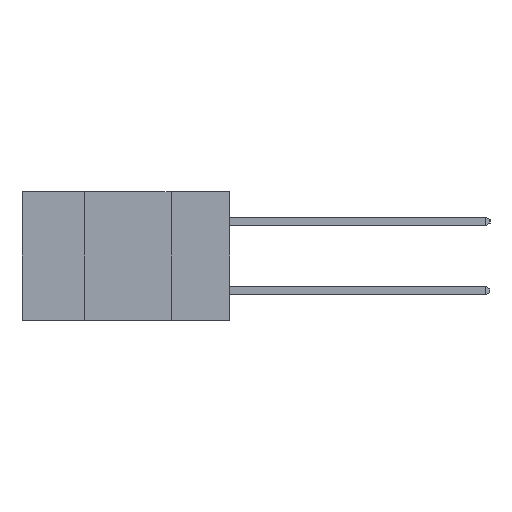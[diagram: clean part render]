
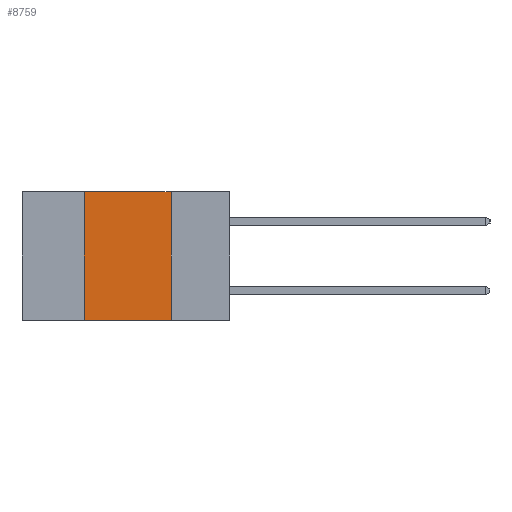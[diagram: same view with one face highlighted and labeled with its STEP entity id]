
A CAD part, left-side view. The second image highlights one B-rep face of the part: STEP entity #8759.
In plain terms, the highlighted planar face has unit normal (-1, 0, 0).
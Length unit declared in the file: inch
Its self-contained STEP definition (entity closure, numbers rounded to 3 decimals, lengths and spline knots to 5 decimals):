
#1374 = EDGE_CURVE ( 'NONE', #15556, #14151, #3866, .T. ) ;
#1461 = DIRECTION ( 'NONE',  ( 0., -1., 0. ) ) ;
#1556 = FACE_OUTER_BOUND ( 'NONE', #8169, .T. ) ;
#2728 = CARTESIAN_POINT ( 'NONE',  ( 0., 0.6, 0. ) ) ;
#2753 = VERTEX_POINT ( 'NONE', #3035 ) ;
#3035 = CARTESIAN_POINT ( 'NONE',  ( 0., 0.42, -0.37 ) ) ;
#3044 = EDGE_CURVE ( 'NONE', #2753, #14151, #6823, .T. ) ;
#3290 = PLANE ( 'NONE',  #7821 ) ;
#3391 = DIRECTION ( 'NONE',  ( 0., -1., 0. ) ) ;
#3539 = VECTOR ( 'NONE', #3391, 39.37008 ) ;
#3866 = LINE ( 'NONE', #14307, #9929 ) ;
#5156 = VERTEX_POINT ( 'NONE', #15204 ) ;
#5336 = ORIENTED_EDGE ( 'NONE', *, *, #3044, .T. ) ;
#5515 = CARTESIAN_POINT ( 'NONE',  ( 0., 0.42, 0. ) ) ;
#6280 = ORIENTED_EDGE ( 'NONE', *, *, #1374, .F. ) ;
#6823 = LINE ( 'NONE', #9938, #3539 ) ;
#7359 = CARTESIAN_POINT ( 'NONE',  ( 0., 0.17, 0. ) ) ;
#7821 = AXIS2_PLACEMENT_3D ( 'NONE', #11954, #9663, #9661 ) ;
#8169 = EDGE_LOOP ( 'NONE', ( #6280, #12516, #11740, #5336 ) ) ;
#8213 = EDGE_CURVE ( 'NONE', #5156, #15556, #11231, .T. ) ;
#8759 = ADVANCED_FACE ( 'NONE', ( #1556 ), #3290, .F. ) ;
#9661 = DIRECTION ( 'NONE',  ( 0., 0., -1. ) ) ;
#9663 = DIRECTION ( 'NONE',  ( 1., 0., 0. ) ) ;
#9929 = VECTOR ( 'NONE', #10033, 39.37008 ) ;
#9938 = CARTESIAN_POINT ( 'NONE',  ( 0., 0.6, -0.37 ) ) ;
#10033 = DIRECTION ( 'NONE',  ( 0., 0., -1. ) ) ;
#11098 = CARTESIAN_POINT ( 'NONE',  ( 0., 0.17, -0.37 ) ) ;
#11231 = LINE ( 'NONE', #2728, #13275 ) ;
#11615 = DIRECTION ( 'NONE',  ( 0., 0., 1. ) ) ;
#11740 = ORIENTED_EDGE ( 'NONE', *, *, #12530, .F. ) ;
#11954 = CARTESIAN_POINT ( 'NONE',  ( 0., 0.6, 0. ) ) ;
#12066 = VECTOR ( 'NONE', #11615, 39.37008 ) ;
#12436 = LINE ( 'NONE', #5515, #12066 ) ;
#12516 = ORIENTED_EDGE ( 'NONE', *, *, #8213, .F. ) ;
#12530 = EDGE_CURVE ( 'NONE', #2753, #5156, #12436, .T. ) ;
#13275 = VECTOR ( 'NONE', #1461, 39.37008 ) ;
#14151 = VERTEX_POINT ( 'NONE', #11098 ) ;
#14307 = CARTESIAN_POINT ( 'NONE',  ( 0., 0.17, 0. ) ) ;
#15204 = CARTESIAN_POINT ( 'NONE',  ( 0., 0.42, 0. ) ) ;
#15556 = VERTEX_POINT ( 'NONE', #7359 ) ;
